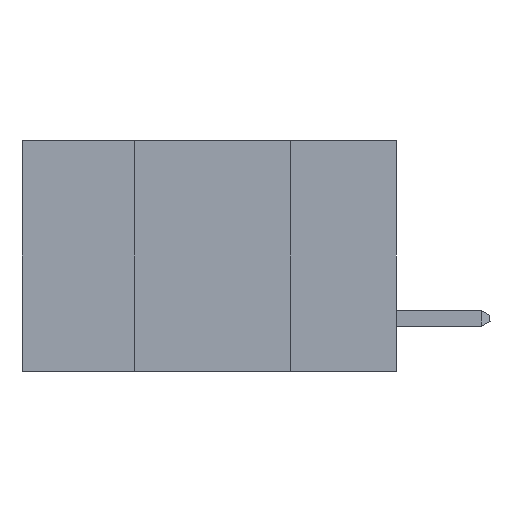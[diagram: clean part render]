
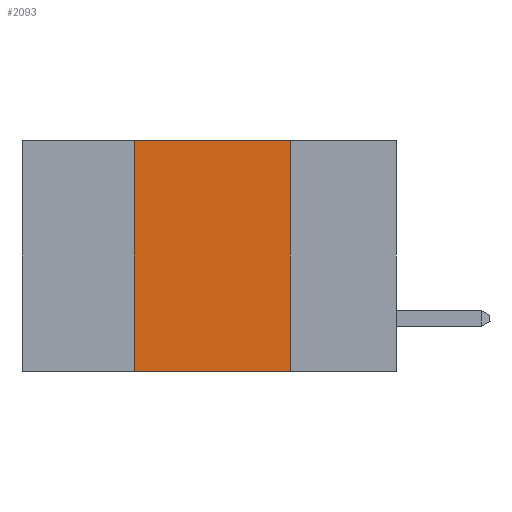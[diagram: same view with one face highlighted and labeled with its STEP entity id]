
A CAD part, left-side view. The second image highlights one B-rep face of the part: STEP entity #2093.
In plain terms, the highlighted planar face has unit normal (-1, 0, 0).
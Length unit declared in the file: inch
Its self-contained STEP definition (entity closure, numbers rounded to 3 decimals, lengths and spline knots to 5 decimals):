
#165 = VECTOR ( 'NONE', #7502, 39.37008 ) ;
#898 = VERTEX_POINT ( 'NONE', #4255 ) ;
#1294 = LINE ( 'NONE', #2178, #11455 ) ;
#1651 = CARTESIAN_POINT ( 'NONE',  ( 0., 0.17, 0. ) ) ;
#1829 = ORIENTED_EDGE ( 'NONE', *, *, #14761, .F. ) ;
#1868 = VERTEX_POINT ( 'NONE', #1651 ) ;
#2093 = ADVANCED_FACE ( 'NONE', ( #19118 ), #4865, .F. ) ;
#2117 = VERTEX_POINT ( 'NONE', #9696 ) ;
#2178 = CARTESIAN_POINT ( 'NONE',  ( 0., 0.42, 0. ) ) ;
#4255 = CARTESIAN_POINT ( 'NONE',  ( 0., 0.42, 0. ) ) ;
#4332 = DIRECTION ( 'NONE',  ( 0., 0., 1. ) ) ;
#4865 = PLANE ( 'NONE',  #16606 ) ;
#5522 = CARTESIAN_POINT ( 'NONE',  ( 0., 0.6, -0.37 ) ) ;
#6976 = DIRECTION ( 'NONE',  ( 0., 0., -1. ) ) ;
#7502 = DIRECTION ( 'NONE',  ( 0., -1., 0. ) ) ;
#7962 = ORIENTED_EDGE ( 'NONE', *, *, #15172, .F. ) ;
#8204 = VECTOR ( 'NONE', #24288, 39.37008 ) ;
#9696 = CARTESIAN_POINT ( 'NONE',  ( 0., 0.17, -0.37 ) ) ;
#11455 = VECTOR ( 'NONE', #4332, 39.37008 ) ;
#12811 = LINE ( 'NONE', #22332, #8204 ) ;
#12836 = VECTOR ( 'NONE', #13219, 39.37008 ) ;
#13219 = DIRECTION ( 'NONE',  ( 0., 0., -1. ) ) ;
#14761 = EDGE_CURVE ( 'NONE', #1868, #2117, #18675, .T. ) ;
#14762 = VERTEX_POINT ( 'NONE', #19154 ) ;
#15172 = EDGE_CURVE ( 'NONE', #898, #1868, #12811, .T. ) ;
#16268 = LINE ( 'NONE', #5522, #165 ) ;
#16606 = AXIS2_PLACEMENT_3D ( 'NONE', #18074, #22050, #6976 ) ;
#18074 = CARTESIAN_POINT ( 'NONE',  ( 0., 0.6, 0. ) ) ;
#18675 = LINE ( 'NONE', #21078, #12836 ) ;
#19118 = FACE_OUTER_BOUND ( 'NONE', #22366, .T. ) ;
#19154 = CARTESIAN_POINT ( 'NONE',  ( 0., 0.42, -0.37 ) ) ;
#19220 = EDGE_CURVE ( 'NONE', #14762, #2117, #16268, .T. ) ;
#21078 = CARTESIAN_POINT ( 'NONE',  ( 0., 0.17, 0. ) ) ;
#22050 = DIRECTION ( 'NONE',  ( 1., 0., 0. ) ) ;
#22332 = CARTESIAN_POINT ( 'NONE',  ( 0., 0.6, 0. ) ) ;
#22366 = EDGE_LOOP ( 'NONE', ( #1829, #7962, #24780, #25386 ) ) ;
#23117 = EDGE_CURVE ( 'NONE', #14762, #898, #1294, .T. ) ;
#24288 = DIRECTION ( 'NONE',  ( 0., -1., 0. ) ) ;
#24780 = ORIENTED_EDGE ( 'NONE', *, *, #23117, .F. ) ;
#25386 = ORIENTED_EDGE ( 'NONE', *, *, #19220, .T. ) ;
